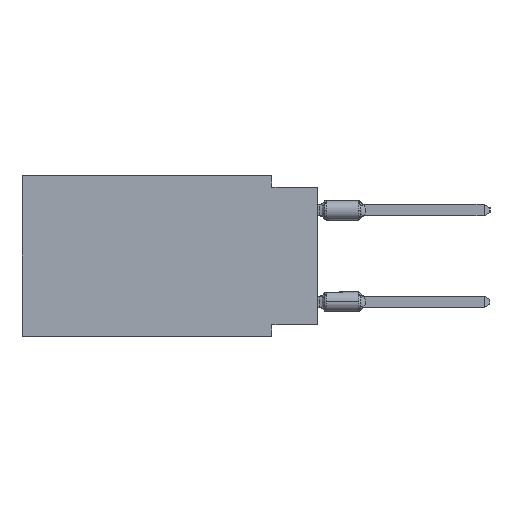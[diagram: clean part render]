
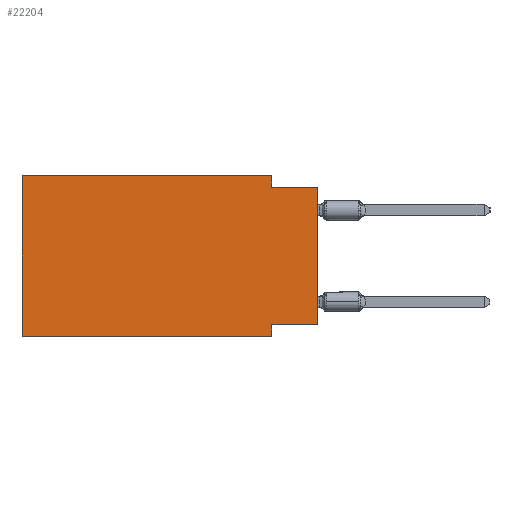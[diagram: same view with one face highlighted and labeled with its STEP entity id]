
A CAD part, left-side view. The second image highlights one B-rep face of the part: STEP entity #22204.
In plain terms, the highlighted planar face has unit normal (-1, 0, 0).
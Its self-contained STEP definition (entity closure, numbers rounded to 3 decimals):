
#619 = CARTESIAN_POINT ( 'NONE',  ( 0., 2.54, -8.89 ) ) ;
#941 = VERTEX_POINT ( 'NONE', #13790 ) ;
#2246 = EDGE_CURVE ( 'NONE', #4276, #25430, #5694, .T. ) ;
#3785 = ORIENTED_EDGE ( 'NONE', *, *, #26342, .F. ) ;
#4276 = VERTEX_POINT ( 'NONE', #24232 ) ;
#5194 = CARTESIAN_POINT ( 'NONE',  ( 0., 16.383, 0. ) ) ;
#5694 = LINE ( 'NONE', #8982, #30787 ) ;
#6113 = CARTESIAN_POINT ( 'NONE',  ( 0., 0., -0.635 ) ) ;
#6335 = VERTEX_POINT ( 'NONE', #6113 ) ;
#7030 = EDGE_CURVE ( 'NONE', #32005, #36226, #36905, .T. ) ;
#7148 = VERTEX_POINT ( 'NONE', #5194 ) ;
#7227 = ORIENTED_EDGE ( 'NONE', *, *, #38782, .F. ) ;
#8350 = VECTOR ( 'NONE', #22102, 1000. ) ;
#8982 = CARTESIAN_POINT ( 'NONE',  ( 0., 16.383, -8.89 ) ) ;
#9571 = EDGE_CURVE ( 'NONE', #941, #6335, #33031, .T. ) ;
#11742 = CARTESIAN_POINT ( 'NONE',  ( 0., 2.54, 0. ) ) ;
#12902 = CARTESIAN_POINT ( 'NONE',  ( 0., 2.54, 0. ) ) ;
#13166 = EDGE_CURVE ( 'NONE', #32005, #6335, #27721, .T. ) ;
#13419 = ORIENTED_EDGE ( 'NONE', *, *, #7030, .F. ) ;
#13790 = CARTESIAN_POINT ( 'NONE',  ( 0., 2.54, -0.635 ) ) ;
#14320 = DIRECTION ( 'NONE',  ( 0., 0., -1. ) ) ;
#14826 = LINE ( 'NONE', #37301, #35273 ) ;
#15804 = CARTESIAN_POINT ( 'NONE',  ( 0., 0., -8.255 ) ) ;
#16002 = DIRECTION ( 'NONE',  ( 0., 0., -1. ) ) ;
#16856 = CARTESIAN_POINT ( 'NONE',  ( 0., 0., 0. ) ) ;
#17235 = VECTOR ( 'NONE', #39375, 1000. ) ;
#17819 = ORIENTED_EDGE ( 'NONE', *, *, #24226, .F. ) ;
#17825 = VECTOR ( 'NONE', #16002, 1000. ) ;
#18506 = VECTOR ( 'NONE', #36868, 1000. ) ;
#19006 = ORIENTED_EDGE ( 'NONE', *, *, #9571, .F. ) ;
#19516 = DIRECTION ( 'NONE',  ( 0., 0., 1. ) ) ;
#20666 = FACE_OUTER_BOUND ( 'NONE', #20890, .T. ) ;
#20890 = EDGE_LOOP ( 'NONE', ( #22364, #19006, #26331, #3785, #7227, #39619, #17819, #13419 ) ) ;
#21280 = VERTEX_POINT ( 'NONE', #11742 ) ;
#21451 = DIRECTION ( 'NONE',  ( 0., -1., 0. ) ) ;
#21856 = CARTESIAN_POINT ( 'NONE',  ( 0., 2.54, -8.255 ) ) ;
#22102 = DIRECTION ( 'NONE',  ( 0., 0., -1. ) ) ;
#22204 = ADVANCED_FACE ( 'NONE', ( #20666 ), #38864, .F. ) ;
#22364 = ORIENTED_EDGE ( 'NONE', *, *, #13166, .T. ) ;
#24226 = EDGE_CURVE ( 'NONE', #36226, #25430, #35030, .T. ) ;
#24232 = CARTESIAN_POINT ( 'NONE',  ( 0., 16.383, -8.89 ) ) ;
#24384 = CARTESIAN_POINT ( 'NONE',  ( 0., 16.383, 0. ) ) ;
#25430 = VERTEX_POINT ( 'NONE', #30640 ) ;
#26331 = ORIENTED_EDGE ( 'NONE', *, *, #34598, .F. ) ;
#26342 = EDGE_CURVE ( 'NONE', #7148, #21280, #30332, .T. ) ;
#26509 = VECTOR ( 'NONE', #19516, 1000. ) ;
#26598 = CARTESIAN_POINT ( 'NONE',  ( 0., 16.383, 0. ) ) ;
#27261 = AXIS2_PLACEMENT_3D ( 'NONE', #26598, #39477, #14320 ) ;
#27309 = DIRECTION ( 'NONE',  ( 0., 0., 1. ) ) ;
#27500 = CARTESIAN_POINT ( 'NONE',  ( 0., 0., -8.255 ) ) ;
#27721 = LINE ( 'NONE', #16856, #26509 ) ;
#30145 = CARTESIAN_POINT ( 'NONE',  ( 0., 0., -0.635 ) ) ;
#30332 = LINE ( 'NONE', #24384, #18506 ) ;
#30640 = CARTESIAN_POINT ( 'NONE',  ( 0., 2.54, -8.89 ) ) ;
#30787 = VECTOR ( 'NONE', #21451, 1000. ) ;
#32005 = VERTEX_POINT ( 'NONE', #15804 ) ;
#33031 = LINE ( 'NONE', #30145, #33650 ) ;
#33650 = VECTOR ( 'NONE', #36480, 1000. ) ;
#34398 = LINE ( 'NONE', #12902, #8350 ) ;
#34598 = EDGE_CURVE ( 'NONE', #21280, #941, #34398, .T. ) ;
#35030 = LINE ( 'NONE', #619, #17825 ) ;
#35273 = VECTOR ( 'NONE', #27309, 1000. ) ;
#36226 = VERTEX_POINT ( 'NONE', #21856 ) ;
#36480 = DIRECTION ( 'NONE',  ( 0., -1., 0. ) ) ;
#36868 = DIRECTION ( 'NONE',  ( 0., -1., 0. ) ) ;
#36905 = LINE ( 'NONE', #27500, #17235 ) ;
#37301 = CARTESIAN_POINT ( 'NONE',  ( 0., 16.383, 0. ) ) ;
#38782 = EDGE_CURVE ( 'NONE', #4276, #7148, #14826, .T. ) ;
#38864 = PLANE ( 'NONE',  #27261 ) ;
#39375 = DIRECTION ( 'NONE',  ( 0., 1., 0. ) ) ;
#39477 = DIRECTION ( 'NONE',  ( 1., 0., 0. ) ) ;
#39619 = ORIENTED_EDGE ( 'NONE', *, *, #2246, .T. ) ;
